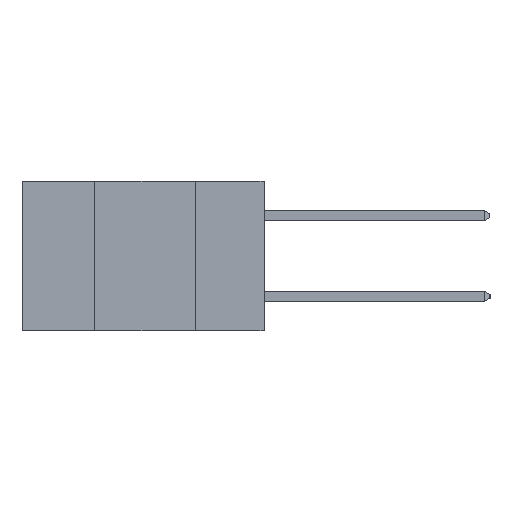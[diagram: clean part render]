
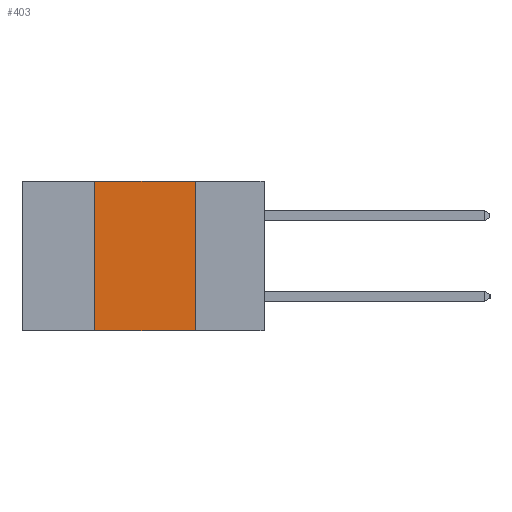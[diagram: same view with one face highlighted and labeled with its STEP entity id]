
A CAD part, left-side view. The second image highlights one B-rep face of the part: STEP entity #403.
In plain terms, the highlighted planar face has unit normal (-1, 0, 0).
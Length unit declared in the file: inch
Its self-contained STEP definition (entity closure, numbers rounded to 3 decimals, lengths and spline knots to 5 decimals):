
#251 = VERTEX_POINT ( 'NONE', #16279 ) ;
#403 = ADVANCED_FACE ( 'NONE', ( #3866 ), #8387, .F. ) ;
#1185 = EDGE_CURVE ( 'NONE', #19224, #3421, #8093, .T. ) ;
#1187 = ORIENTED_EDGE ( 'NONE', *, *, #5996, .F. ) ;
#1437 = CARTESIAN_POINT ( 'NONE',  ( 0., 0.17, 0. ) ) ;
#1567 = VECTOR ( 'NONE', #9641, 39.37008 ) ;
#1823 = CARTESIAN_POINT ( 'NONE',  ( 0., 0.6, 0. ) ) ;
#2072 = DIRECTION ( 'NONE',  ( 0., 0., 1. ) ) ;
#2323 = LINE ( 'NONE', #2888, #15557 ) ;
#2888 = CARTESIAN_POINT ( 'NONE',  ( 0., 0.6, -0.37 ) ) ;
#3421 = VERTEX_POINT ( 'NONE', #1437 ) ;
#3866 = FACE_OUTER_BOUND ( 'NONE', #18696, .T. ) ;
#4012 = VERTEX_POINT ( 'NONE', #10700 ) ;
#5996 = EDGE_CURVE ( 'NONE', #3421, #251, #10134, .T. ) ;
#7606 = VECTOR ( 'NONE', #13186, 39.37008 ) ;
#8032 = CARTESIAN_POINT ( 'NONE',  ( 0., 0.17, -0.37 ) ) ;
#8093 = LINE ( 'NONE', #11780, #7606 ) ;
#8135 = LINE ( 'NONE', #13273, #19805 ) ;
#8387 = PLANE ( 'NONE',  #17187 ) ;
#9463 = ORIENTED_EDGE ( 'NONE', *, *, #1185, .F. ) ;
#9641 = DIRECTION ( 'NONE',  ( 0., 0., -1. ) ) ;
#10134 = LINE ( 'NONE', #8032, #1567 ) ;
#10700 = CARTESIAN_POINT ( 'NONE',  ( 0., 0.42, -0.37 ) ) ;
#11780 = CARTESIAN_POINT ( 'NONE',  ( 0., 0.6, 0. ) ) ;
#13123 = EDGE_CURVE ( 'NONE', #4012, #19224, #8135, .T. ) ;
#13186 = DIRECTION ( 'NONE',  ( 0., -1., 0. ) ) ;
#13273 = CARTESIAN_POINT ( 'NONE',  ( 0., 0.42, -0.37 ) ) ;
#13790 = CARTESIAN_POINT ( 'NONE',  ( 0., 0.42, 0. ) ) ;
#14037 = DIRECTION ( 'NONE',  ( 0., -1., 0. ) ) ;
#14478 = DIRECTION ( 'NONE',  ( 0., 0., -1. ) ) ;
#14598 = EDGE_CURVE ( 'NONE', #4012, #251, #2323, .T. ) ;
#15557 = VECTOR ( 'NONE', #14037, 39.37008 ) ;
#16279 = CARTESIAN_POINT ( 'NONE',  ( 0., 0.17, -0.37 ) ) ;
#17118 = ORIENTED_EDGE ( 'NONE', *, *, #13123, .F. ) ;
#17187 = AXIS2_PLACEMENT_3D ( 'NONE', #1823, #20127, #14478 ) ;
#18508 = ORIENTED_EDGE ( 'NONE', *, *, #14598, .T. ) ;
#18696 = EDGE_LOOP ( 'NONE', ( #1187, #9463, #17118, #18508 ) ) ;
#19224 = VERTEX_POINT ( 'NONE', #13790 ) ;
#19805 = VECTOR ( 'NONE', #2072, 39.37008 ) ;
#20127 = DIRECTION ( 'NONE',  ( 1., 0., 0. ) ) ;
